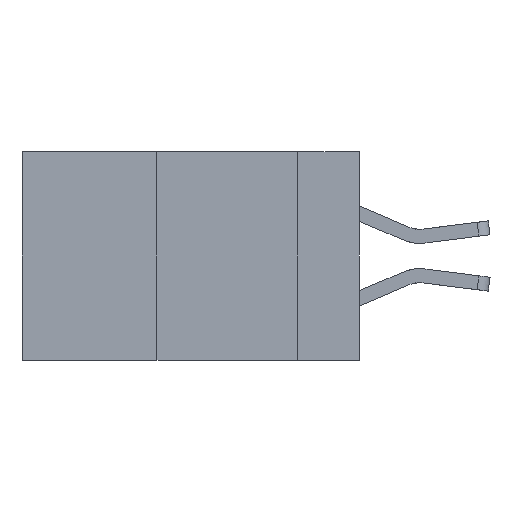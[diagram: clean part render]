
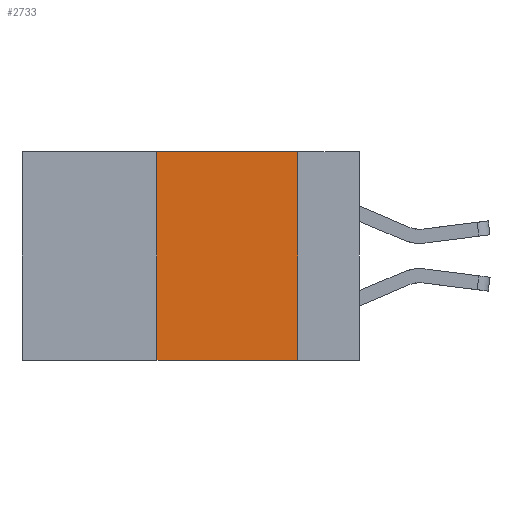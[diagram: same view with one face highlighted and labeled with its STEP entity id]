
A CAD part, left-side view. The second image highlights one B-rep face of the part: STEP entity #2733.
In plain terms, the highlighted planar face has unit normal (-1, 0, 0).
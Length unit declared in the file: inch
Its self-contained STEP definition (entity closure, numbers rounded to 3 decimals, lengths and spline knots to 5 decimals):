
#355 = CARTESIAN_POINT ( 'NONE',  ( 0., 0.11, -0.37 ) ) ;
#367 = CARTESIAN_POINT ( 'NONE',  ( 0., 0.6, 0. ) ) ;
#519 = EDGE_LOOP ( 'NONE', ( #3875, #3142, #2924, #8592 ) ) ;
#614 = CARTESIAN_POINT ( 'NONE',  ( 0., 0.11, 0. ) ) ;
#874 = EDGE_CURVE ( 'NONE', #8945, #2121, #2016, .T. ) ;
#1510 = VECTOR ( 'NONE', #3435, 39.37008 ) ;
#1662 = EDGE_CURVE ( 'NONE', #2121, #7241, #3458, .T. ) ;
#1839 = AXIS2_PLACEMENT_3D ( 'NONE', #367, #2507, #9011 ) ;
#2016 = LINE ( 'NONE', #9216, #5444 ) ;
#2103 = VECTOR ( 'NONE', #2589, 39.37008 ) ;
#2121 = VERTEX_POINT ( 'NONE', #3362 ) ;
#2477 = DIRECTION ( 'NONE',  ( 0., -1., 0. ) ) ;
#2507 = DIRECTION ( 'NONE',  ( 1., 0., 0. ) ) ;
#2539 = PLANE ( 'NONE',  #1839 ) ;
#2589 = DIRECTION ( 'NONE',  ( 0., 0., -1. ) ) ;
#2733 = ADVANCED_FACE ( 'NONE', ( #7222 ), #2539, .F. ) ;
#2919 = EDGE_CURVE ( 'NONE', #7241, #8788, #5505, .T. ) ;
#2924 = ORIENTED_EDGE ( 'NONE', *, *, #874, .F. ) ;
#3142 = ORIENTED_EDGE ( 'NONE', *, *, #1662, .F. ) ;
#3362 = CARTESIAN_POINT ( 'NONE',  ( 0., 0.36, 0. ) ) ;
#3435 = DIRECTION ( 'NONE',  ( 0., -1., 0. ) ) ;
#3458 = LINE ( 'NONE', #3536, #1510 ) ;
#3536 = CARTESIAN_POINT ( 'NONE',  ( 0., 0.6, 0. ) ) ;
#3875 = ORIENTED_EDGE ( 'NONE', *, *, #2919, .F. ) ;
#4093 = DIRECTION ( 'NONE',  ( 0., 0., 1. ) ) ;
#4437 = VECTOR ( 'NONE', #2477, 39.37008 ) ;
#4484 = CARTESIAN_POINT ( 'NONE',  ( 0., 0.36, -0.37 ) ) ;
#4672 = LINE ( 'NONE', #5075, #4437 ) ;
#5075 = CARTESIAN_POINT ( 'NONE',  ( 0., 0.6, -0.37 ) ) ;
#5444 = VECTOR ( 'NONE', #4093, 39.37008 ) ;
#5505 = LINE ( 'NONE', #614, #2103 ) ;
#7222 = FACE_OUTER_BOUND ( 'NONE', #519, .T. ) ;
#7241 = VERTEX_POINT ( 'NONE', #7405 ) ;
#7401 = EDGE_CURVE ( 'NONE', #8945, #8788, #4672, .T. ) ;
#7405 = CARTESIAN_POINT ( 'NONE',  ( 0., 0.11, 0. ) ) ;
#8592 = ORIENTED_EDGE ( 'NONE', *, *, #7401, .T. ) ;
#8788 = VERTEX_POINT ( 'NONE', #355 ) ;
#8945 = VERTEX_POINT ( 'NONE', #4484 ) ;
#9011 = DIRECTION ( 'NONE',  ( 0., 0., -1. ) ) ;
#9216 = CARTESIAN_POINT ( 'NONE',  ( 0., 0.36, 0. ) ) ;
